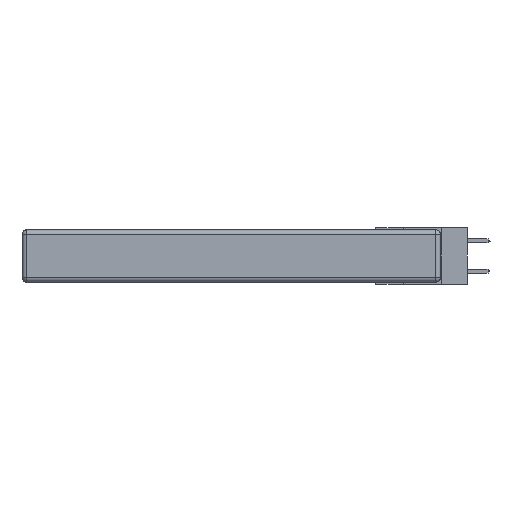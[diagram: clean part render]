
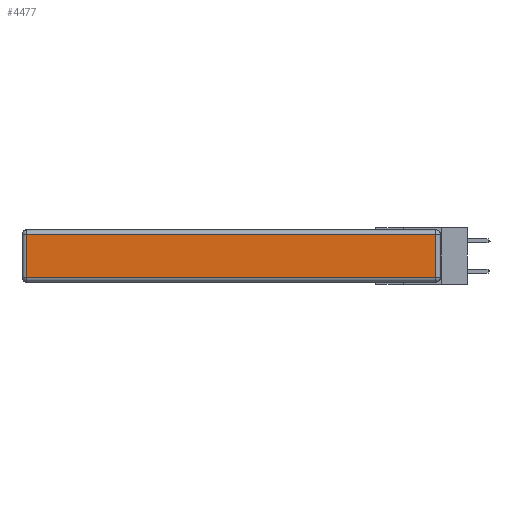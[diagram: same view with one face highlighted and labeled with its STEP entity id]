
A CAD part, left-side view. The second image highlights one B-rep face of the part: STEP entity #4477.
In plain terms, the highlighted planar face has unit normal (-1, 0, 0).
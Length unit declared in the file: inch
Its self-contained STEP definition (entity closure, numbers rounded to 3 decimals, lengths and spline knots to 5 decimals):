
#102 = VECTOR ( 'NONE', #7573, 39.37008 ) ;
#776 = VECTOR ( 'NONE', #11296, 39.37008 ) ;
#1926 = EDGE_LOOP ( 'NONE', ( #17938, #12609, #9357, #16833 ) ) ;
#1965 = LINE ( 'NONE', #3793, #776 ) ;
#2138 = CARTESIAN_POINT ( 'NONE',  ( 0., 0.03, -0.313 ) ) ;
#2159 = VECTOR ( 'NONE', #6554, 39.37008 ) ;
#2669 = VERTEX_POINT ( 'NONE', #9749 ) ;
#2678 = EDGE_CURVE ( 'NONE', #8875, #2669, #1965, .T. ) ;
#3793 = CARTESIAN_POINT ( 'NONE',  ( 0., 2.72, -0.343 ) ) ;
#4477 = ADVANCED_FACE ( 'NONE', ( #14390 ), #18054, .T. ) ;
#4860 = AXIS2_PLACEMENT_3D ( 'NONE', #5881, #16447, #17934 ) ;
#5400 = EDGE_CURVE ( 'NONE', #17354, #8875, #19387, .T. ) ;
#5881 = CARTESIAN_POINT ( 'NONE',  ( 0., 0., -0.343 ) ) ;
#6554 = DIRECTION ( 'NONE',  ( 0., -1., 0. ) ) ;
#7573 = DIRECTION ( 'NONE',  ( 0., 0., 1. ) ) ;
#8312 = EDGE_CURVE ( 'NONE', #2669, #18951, #10111, .T. ) ;
#8558 = VECTOR ( 'NONE', #14452, 39.37008 ) ;
#8875 = VERTEX_POINT ( 'NONE', #17226 ) ;
#9357 = ORIENTED_EDGE ( 'NONE', *, *, #5400, .T. ) ;
#9749 = CARTESIAN_POINT ( 'NONE',  ( 0., 2.72, -0.313 ) ) ;
#9988 = CARTESIAN_POINT ( 'NONE',  ( 0., 2.75, -0.03 ) ) ;
#10111 = LINE ( 'NONE', #17493, #2159 ) ;
#11145 = CARTESIAN_POINT ( 'NONE',  ( 0., 0.03, -0.03 ) ) ;
#11296 = DIRECTION ( 'NONE',  ( 0., 0., -1. ) ) ;
#12609 = ORIENTED_EDGE ( 'NONE', *, *, #14174, .T. ) ;
#14174 = EDGE_CURVE ( 'NONE', #18951, #17354, #16302, .T. ) ;
#14390 = FACE_OUTER_BOUND ( 'NONE', #1926, .T. ) ;
#14452 = DIRECTION ( 'NONE',  ( 0., 1., 0. ) ) ;
#15256 = CARTESIAN_POINT ( 'NONE',  ( 0., 0.03, -0.343 ) ) ;
#16302 = LINE ( 'NONE', #15256, #102 ) ;
#16447 = DIRECTION ( 'NONE',  ( -1., 0., 0. ) ) ;
#16833 = ORIENTED_EDGE ( 'NONE', *, *, #2678, .T. ) ;
#17226 = CARTESIAN_POINT ( 'NONE',  ( 0., 2.72, -0.03 ) ) ;
#17354 = VERTEX_POINT ( 'NONE', #11145 ) ;
#17493 = CARTESIAN_POINT ( 'NONE',  ( 0., 0., -0.313 ) ) ;
#17934 = DIRECTION ( 'NONE',  ( 0., 0., 1. ) ) ;
#17938 = ORIENTED_EDGE ( 'NONE', *, *, #8312, .T. ) ;
#18054 = PLANE ( 'NONE',  #4860 ) ;
#18951 = VERTEX_POINT ( 'NONE', #2138 ) ;
#19387 = LINE ( 'NONE', #9988, #8558 ) ;
